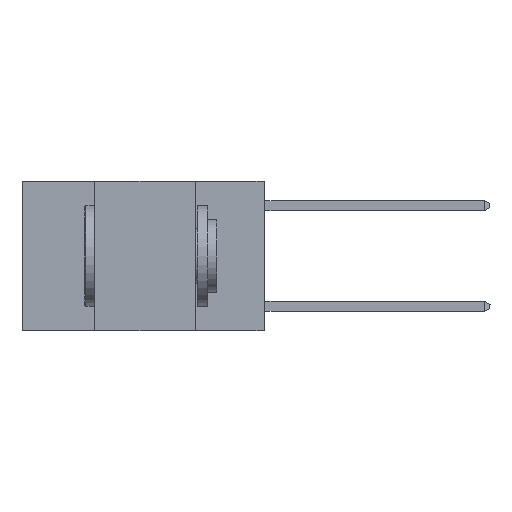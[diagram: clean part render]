
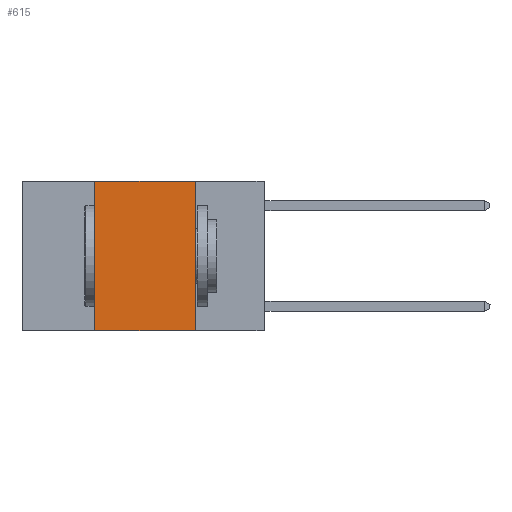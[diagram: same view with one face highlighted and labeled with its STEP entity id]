
A CAD part, left-side view. The second image highlights one B-rep face of the part: STEP entity #615.
In plain terms, the highlighted planar face has unit normal (-1, 0, 0).
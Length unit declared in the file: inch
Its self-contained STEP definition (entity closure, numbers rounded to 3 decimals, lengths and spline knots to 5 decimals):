
#197 = ORIENTED_EDGE ( 'NONE', *, *, #14074, .T. ) ;
#615 = ADVANCED_FACE ( 'NONE', ( #13707 ), #12336, .F. ) ;
#715 = CARTESIAN_POINT ( 'NONE',  ( 0., 0.42, -0.37 ) ) ;
#1321 = EDGE_CURVE ( 'NONE', #12319, #17521, #1358, .T. ) ;
#1358 = LINE ( 'NONE', #1673, #9597 ) ;
#1673 = CARTESIAN_POINT ( 'NONE',  ( 0., 0.42, 0. ) ) ;
#1937 = CARTESIAN_POINT ( 'NONE',  ( 0., 0.6, 0. ) ) ;
#2208 = ORIENTED_EDGE ( 'NONE', *, *, #1321, .F. ) ;
#2246 = DIRECTION ( 'NONE',  ( 0., 0., -1. ) ) ;
#2274 = DIRECTION ( 'NONE',  ( 1., 0., 0. ) ) ;
#2619 = VECTOR ( 'NONE', #19696, 39.37008 ) ;
#3518 = CARTESIAN_POINT ( 'NONE',  ( 0., 0.6, 0. ) ) ;
#4659 = CARTESIAN_POINT ( 'NONE',  ( 0., 0.6, -0.37 ) ) ;
#5049 = DIRECTION ( 'NONE',  ( 0., 0., -1. ) ) ;
#5563 = VERTEX_POINT ( 'NONE', #14035 ) ;
#5846 = EDGE_CURVE ( 'NONE', #15331, #5563, #16922, .T. ) ;
#6721 = LINE ( 'NONE', #4659, #10975 ) ;
#7837 = ORIENTED_EDGE ( 'NONE', *, *, #5846, .F. ) ;
#9597 = VECTOR ( 'NONE', #10291, 39.37008 ) ;
#10291 = DIRECTION ( 'NONE',  ( 0., 0., 1. ) ) ;
#10809 = EDGE_LOOP ( 'NONE', ( #7837, #13890, #2208, #197 ) ) ;
#10975 = VECTOR ( 'NONE', #14257, 39.37008 ) ;
#11216 = LINE ( 'NONE', #1937, #2619 ) ;
#11481 = CARTESIAN_POINT ( 'NONE',  ( 0., 0.17, 0. ) ) ;
#12319 = VERTEX_POINT ( 'NONE', #715 ) ;
#12336 = PLANE ( 'NONE',  #13437 ) ;
#12645 = VECTOR ( 'NONE', #5049, 39.37008 ) ;
#13437 = AXIS2_PLACEMENT_3D ( 'NONE', #3518, #2274, #2246 ) ;
#13707 = FACE_OUTER_BOUND ( 'NONE', #10809, .T. ) ;
#13890 = ORIENTED_EDGE ( 'NONE', *, *, #19402, .F. ) ;
#14035 = CARTESIAN_POINT ( 'NONE',  ( 0., 0.17, -0.37 ) ) ;
#14074 = EDGE_CURVE ( 'NONE', #12319, #5563, #6721, .T. ) ;
#14257 = DIRECTION ( 'NONE',  ( 0., -1., 0. ) ) ;
#15331 = VERTEX_POINT ( 'NONE', #11481 ) ;
#16922 = LINE ( 'NONE', #17792, #12645 ) ;
#17521 = VERTEX_POINT ( 'NONE', #17912 ) ;
#17792 = CARTESIAN_POINT ( 'NONE',  ( 0., 0.17, 0. ) ) ;
#17912 = CARTESIAN_POINT ( 'NONE',  ( 0., 0.42, 0. ) ) ;
#19402 = EDGE_CURVE ( 'NONE', #17521, #15331, #11216, .T. ) ;
#19696 = DIRECTION ( 'NONE',  ( 0., -1., 0. ) ) ;
